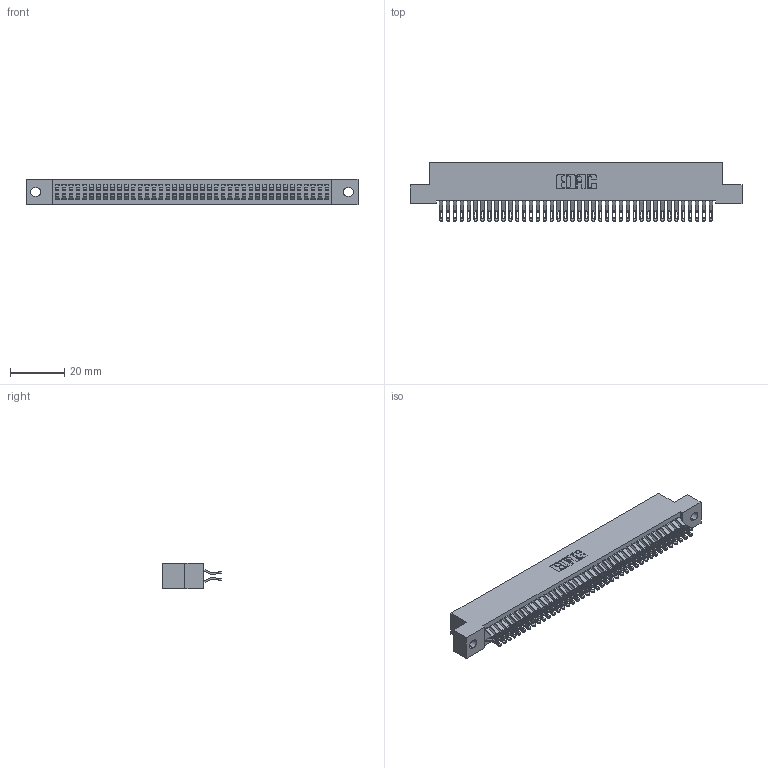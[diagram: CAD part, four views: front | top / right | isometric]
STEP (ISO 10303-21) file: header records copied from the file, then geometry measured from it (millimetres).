
FILE_DESCRIPTION (( 'STEP AP203' ), '1' );
FILE_NAME ('342-080-555-202.STEP', '2019-10-04T11:46:03', ( '' ), ( '' ), 'SwSTEP 2.0', 'SolidWorks 2016', '' );
FILE_SCHEMA (( 'CONFIG_CONTROL_DESIGN' ));
Length unit declared in the file: inch
Products named in the file (3): 345-292-001_555 Tail; 342-080-555-202; 342 Part_.128 Slot
Assembly tree (81 placements, depth 2):
  342-080-555-202
    342 Part_.128 Slot
    345-292-001_555 Tail  x80
Bounding box: 121.92 x 21.47 x 9.4 mm (x, y, z)
Volume: 11115.2 mm3; surface area: 18577 mm2
Topology: 81 solids, 81 shells, 4754 faces, 14951 edges, 9966 vertices
Faces by surface type: plane 2790, cylinder 1964
Entity records: 26321 total; most frequent: CARTESIAN_POINT 4400, ORIENTED_EDGE 4306, DIRECTION 3733, EDGE_CURVE 2153, VECTOR 2005, LINE 2005, VERTEX_POINT 1434, AXIS2_PLACEMENT_3D 864
